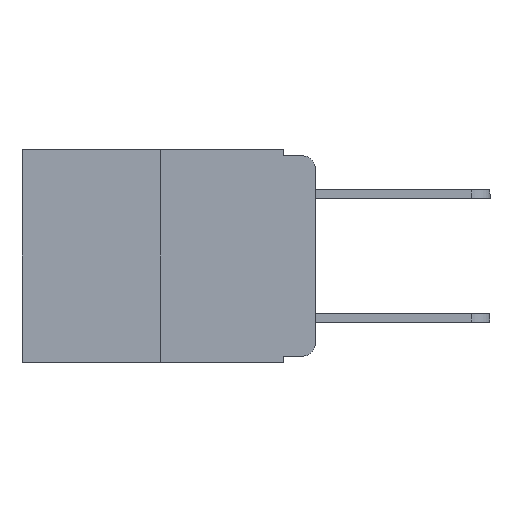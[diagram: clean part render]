
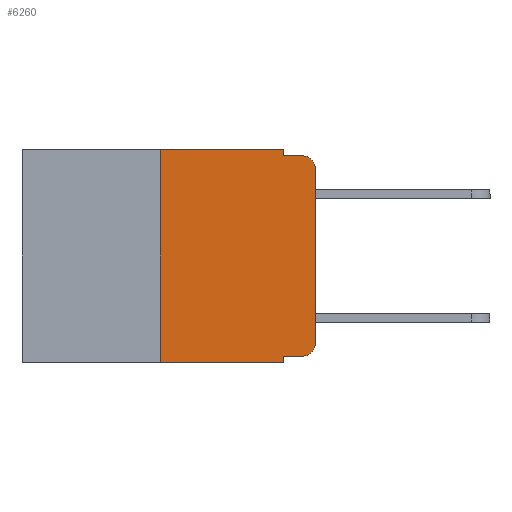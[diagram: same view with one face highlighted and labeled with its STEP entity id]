
A CAD part, left-side view. The second image highlights one B-rep face of the part: STEP entity #6260.
In plain terms, the highlighted planar face has unit normal (-1, 0, 0).
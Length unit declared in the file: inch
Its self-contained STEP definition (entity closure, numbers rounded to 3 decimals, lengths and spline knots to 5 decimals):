
#20 = EDGE_CURVE ( 'NONE', #6707, #522, #9331, .T. ) ;
#228 = DIRECTION ( 'NONE',  ( 0., 0., -1. ) ) ;
#314 = CARTESIAN_POINT ( 'NONE',  ( 0., 0., 0. ) ) ;
#366 = ORIENTED_EDGE ( 'NONE', *, *, #14250, .T. ) ;
#522 = VERTEX_POINT ( 'NONE', #22645 ) ;
#1053 = ORIENTED_EDGE ( 'NONE', *, *, #7729, .F. ) ;
#1097 = VERTEX_POINT ( 'NONE', #15918 ) ;
#2454 = LINE ( 'NONE', #5861, #19182 ) ;
#2642 = VERTEX_POINT ( 'NONE', #16730 ) ;
#2663 = LINE ( 'NONE', #22619, #20064 ) ;
#2720 = VECTOR ( 'NONE', #15530, 39.37008 ) ;
#2771 = EDGE_CURVE ( 'NONE', #2642, #15244, #3667, .T. ) ;
#3199 = DIRECTION ( 'NONE',  ( 0., 0., -1. ) ) ;
#3667 = LINE ( 'NONE', #19519, #13897 ) ;
#3762 = DIRECTION ( 'NONE',  ( 0., 0., 1. ) ) ;
#4497 = AXIS2_PLACEMENT_3D ( 'NONE', #22856, #6785, #21095 ) ;
#4730 = EDGE_CURVE ( 'NONE', #9966, #15560, #2454, .T. ) ;
#4759 = ORIENTED_EDGE ( 'NONE', *, *, #20, .T. ) ;
#5372 = AXIS2_PLACEMENT_3D ( 'NONE', #11446, #5932, #16500 ) ;
#5703 = DIRECTION ( 'NONE',  ( 0., 0., -1. ) ) ;
#5735 = EDGE_CURVE ( 'NONE', #13217, #6625, #12120, .T. ) ;
#5773 = CARTESIAN_POINT ( 'NONE',  ( 0., 0.051, -0.333 ) ) ;
#5861 = CARTESIAN_POINT ( 'NONE',  ( 0., 0.051, -0.333 ) ) ;
#5932 = DIRECTION ( 'NONE',  ( -1., 0., 0. ) ) ;
#6260 = ADVANCED_FACE ( 'NONE', ( #17581 ), #8786, .F. ) ;
#6625 = VERTEX_POINT ( 'NONE', #6764 ) ;
#6707 = VERTEX_POINT ( 'NONE', #19557 ) ;
#6764 = CARTESIAN_POINT ( 'NONE',  ( 0., 0.051, 0. ) ) ;
#6785 = DIRECTION ( 'NONE',  ( -1., 0., 0. ) ) ;
#7724 = EDGE_CURVE ( 'NONE', #15560, #6707, #16974, .T. ) ;
#7729 = EDGE_CURVE ( 'NONE', #6625, #1097, #13089, .T. ) ;
#8369 = AXIS2_PLACEMENT_3D ( 'NONE', #14175, #8910, #228 ) ;
#8371 = CARTESIAN_POINT ( 'NONE',  ( 0., 0.473, 0. ) ) ;
#8786 = PLANE ( 'NONE',  #8369 ) ;
#8910 = DIRECTION ( 'NONE',  ( 1., 0., 0. ) ) ;
#9331 = LINE ( 'NONE', #314, #19237 ) ;
#9607 = DIRECTION ( 'NONE',  ( 0., -1., 0. ) ) ;
#9626 = EDGE_CURVE ( 'NONE', #9966, #15244, #17163, .T. ) ;
#9903 = EDGE_LOOP ( 'NONE', ( #4759, #366, #15333, #1053, #12562, #19087, #16659, #10807, #12037, #12095 ) ) ;
#9966 = VERTEX_POINT ( 'NONE', #5773 ) ;
#10807 = ORIENTED_EDGE ( 'NONE', *, *, #9626, .F. ) ;
#11446 = CARTESIAN_POINT ( 'NONE',  ( 0., 0.02, -0.313 ) ) ;
#12037 = ORIENTED_EDGE ( 'NONE', *, *, #4730, .T. ) ;
#12095 = ORIENTED_EDGE ( 'NONE', *, *, #7724, .T. ) ;
#12120 = LINE ( 'NONE', #8371, #2720 ) ;
#12187 = CARTESIAN_POINT ( 'NONE',  ( 0., 0.02, -0.333 ) ) ;
#12189 = VECTOR ( 'NONE', #3199, 39.37008 ) ;
#12463 = DIRECTION ( 'NONE',  ( 0., -1., 0. ) ) ;
#12562 = ORIENTED_EDGE ( 'NONE', *, *, #5735, .F. ) ;
#12923 = LINE ( 'NONE', #19855, #14084 ) ;
#13089 = LINE ( 'NONE', #18361, #15854 ) ;
#13217 = VERTEX_POINT ( 'NONE', #22244 ) ;
#13897 = VECTOR ( 'NONE', #12463, 39.37008 ) ;
#14084 = VECTOR ( 'NONE', #3762, 39.37008 ) ;
#14175 = CARTESIAN_POINT ( 'NONE',  ( 0., 0.473, 0. ) ) ;
#14250 = EDGE_CURVE ( 'NONE', #522, #19986, #19112, .T. ) ;
#15244 = VERTEX_POINT ( 'NONE', #15995 ) ;
#15333 = ORIENTED_EDGE ( 'NONE', *, *, #22965, .F. ) ;
#15530 = DIRECTION ( 'NONE',  ( 0., -1., 0. ) ) ;
#15560 = VERTEX_POINT ( 'NONE', #12187 ) ;
#15854 = VECTOR ( 'NONE', #5703, 39.37008 ) ;
#15918 = CARTESIAN_POINT ( 'NONE',  ( 0., 0.051, -0.01 ) ) ;
#15995 = CARTESIAN_POINT ( 'NONE',  ( 0., 0.051, -0.343 ) ) ;
#16030 = CARTESIAN_POINT ( 'NONE',  ( 0., 0.02, -0.01 ) ) ;
#16500 = DIRECTION ( 'NONE',  ( 0., 0., -1. ) ) ;
#16659 = ORIENTED_EDGE ( 'NONE', *, *, #2771, .T. ) ;
#16730 = CARTESIAN_POINT ( 'NONE',  ( 0., 0.25, -0.343 ) ) ;
#16974 = CIRCLE ( 'NONE', #5372, 0.02 ) ;
#16981 = DIRECTION ( 'NONE',  ( 0., -1., 0. ) ) ;
#17163 = LINE ( 'NONE', #20924, #12189 ) ;
#17581 = FACE_OUTER_BOUND ( 'NONE', #9903, .T. ) ;
#18361 = CARTESIAN_POINT ( 'NONE',  ( 0., 0.051, 0. ) ) ;
#19087 = ORIENTED_EDGE ( 'NONE', *, *, #21102, .F. ) ;
#19112 = CIRCLE ( 'NONE', #4497, 0.02 ) ;
#19182 = VECTOR ( 'NONE', #9607, 39.37008 ) ;
#19237 = VECTOR ( 'NONE', #21673, 39.37008 ) ;
#19519 = CARTESIAN_POINT ( 'NONE',  ( 0., 0.473, -0.343 ) ) ;
#19557 = CARTESIAN_POINT ( 'NONE',  ( 0., 0., -0.313 ) ) ;
#19855 = CARTESIAN_POINT ( 'NONE',  ( 0., 0.25, 0. ) ) ;
#19986 = VERTEX_POINT ( 'NONE', #16030 ) ;
#20064 = VECTOR ( 'NONE', #16981, 39.37008 ) ;
#20924 = CARTESIAN_POINT ( 'NONE',  ( 0., 0.051, 0. ) ) ;
#21095 = DIRECTION ( 'NONE',  ( 0., 0., -1. ) ) ;
#21102 = EDGE_CURVE ( 'NONE', #2642, #13217, #12923, .T. ) ;
#21673 = DIRECTION ( 'NONE',  ( 0., 0., 1. ) ) ;
#22244 = CARTESIAN_POINT ( 'NONE',  ( 0., 0.25, 0. ) ) ;
#22619 = CARTESIAN_POINT ( 'NONE',  ( 0., 0.051, -0.01 ) ) ;
#22645 = CARTESIAN_POINT ( 'NONE',  ( 0., 0., -0.03 ) ) ;
#22856 = CARTESIAN_POINT ( 'NONE',  ( 0., 0.02, -0.03 ) ) ;
#22965 = EDGE_CURVE ( 'NONE', #1097, #19986, #2663, .T. ) ;
